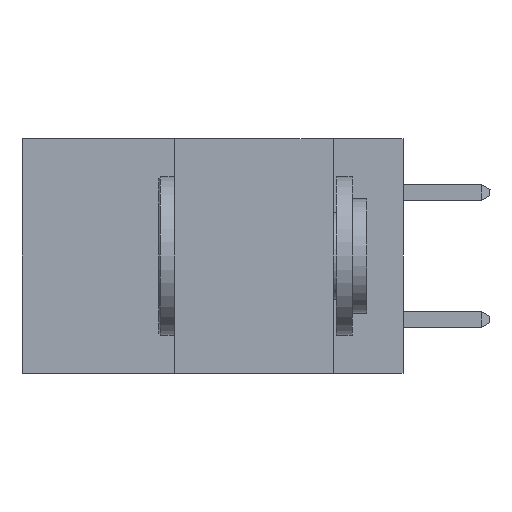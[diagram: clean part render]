
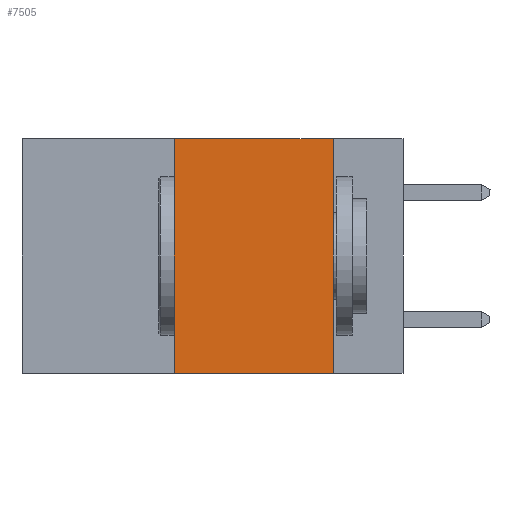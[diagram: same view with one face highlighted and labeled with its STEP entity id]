
A CAD part, left-side view. The second image highlights one B-rep face of the part: STEP entity #7505.
In plain terms, the highlighted planar face has unit normal (-1, 0, 0).
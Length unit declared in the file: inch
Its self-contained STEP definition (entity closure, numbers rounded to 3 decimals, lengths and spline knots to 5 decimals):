
#236 = CARTESIAN_POINT ( 'NONE',  ( 0., 0.36, 0. ) ) ;
#757 = VERTEX_POINT ( 'NONE', #8010 ) ;
#1909 = VERTEX_POINT ( 'NONE', #3314 ) ;
#2344 = FACE_OUTER_BOUND ( 'NONE', #10296, .T. ) ;
#3314 = CARTESIAN_POINT ( 'NONE',  ( 0., 0.11, 0. ) ) ;
#4772 = VERTEX_POINT ( 'NONE', #236 ) ;
#5171 = ORIENTED_EDGE ( 'NONE', *, *, #25024, .F. ) ;
#6212 = DIRECTION ( 'NONE',  ( 0., -1., 0. ) ) ;
#6298 = EDGE_CURVE ( 'NONE', #10347, #4772, #18965, .T. ) ;
#6410 = LINE ( 'NONE', #18036, #16917 ) ;
#6647 = EDGE_CURVE ( 'NONE', #10347, #757, #21959, .T. ) ;
#6810 = CARTESIAN_POINT ( 'NONE',  ( 0., 0.36, -0.37 ) ) ;
#6929 = VECTOR ( 'NONE', #21802, 39.37008 ) ;
#7505 = ADVANCED_FACE ( 'NONE', ( #2344 ), #8264, .F. ) ;
#7858 = VECTOR ( 'NONE', #20821, 39.37008 ) ;
#8010 = CARTESIAN_POINT ( 'NONE',  ( 0., 0.11, -0.37 ) ) ;
#8264 = PLANE ( 'NONE',  #16853 ) ;
#10253 = DIRECTION ( 'NONE',  ( 0., 0., -1. ) ) ;
#10296 = EDGE_LOOP ( 'NONE', ( #20278, #5171, #16296, #21480 ) ) ;
#10347 = VERTEX_POINT ( 'NONE', #6810 ) ;
#11590 = DIRECTION ( 'NONE',  ( 0., 0., -1. ) ) ;
#14985 = CARTESIAN_POINT ( 'NONE',  ( 0., 0.36, 0. ) ) ;
#15986 = EDGE_CURVE ( 'NONE', #1909, #757, #23777, .T. ) ;
#16023 = CARTESIAN_POINT ( 'NONE',  ( 0., 0.6, -0.37 ) ) ;
#16296 = ORIENTED_EDGE ( 'NONE', *, *, #6298, .F. ) ;
#16853 = AXIS2_PLACEMENT_3D ( 'NONE', #23751, #21967, #10253 ) ;
#16917 = VECTOR ( 'NONE', #6212, 39.37008 ) ;
#18036 = CARTESIAN_POINT ( 'NONE',  ( 0., 0.6, 0. ) ) ;
#18743 = VECTOR ( 'NONE', #11590, 39.37008 ) ;
#18965 = LINE ( 'NONE', #14985, #7858 ) ;
#19411 = CARTESIAN_POINT ( 'NONE',  ( 0., 0.11, 0. ) ) ;
#20278 = ORIENTED_EDGE ( 'NONE', *, *, #15986, .F. ) ;
#20821 = DIRECTION ( 'NONE',  ( 0., 0., 1. ) ) ;
#21480 = ORIENTED_EDGE ( 'NONE', *, *, #6647, .T. ) ;
#21802 = DIRECTION ( 'NONE',  ( 0., -1., 0. ) ) ;
#21959 = LINE ( 'NONE', #16023, #6929 ) ;
#21967 = DIRECTION ( 'NONE',  ( 1., 0., 0. ) ) ;
#23751 = CARTESIAN_POINT ( 'NONE',  ( 0., 0.6, 0. ) ) ;
#23777 = LINE ( 'NONE', #19411, #18743 ) ;
#25024 = EDGE_CURVE ( 'NONE', #4772, #1909, #6410, .T. ) ;
